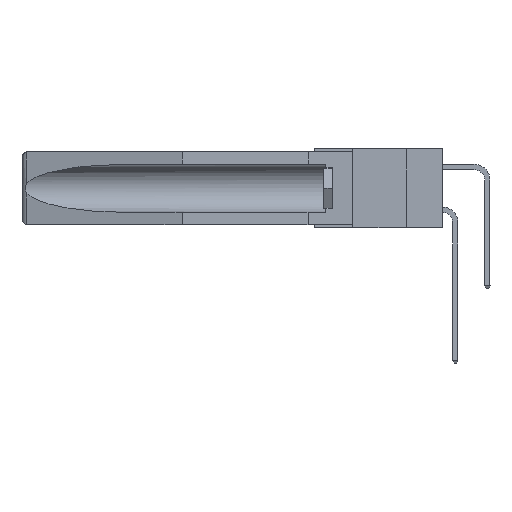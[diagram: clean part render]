
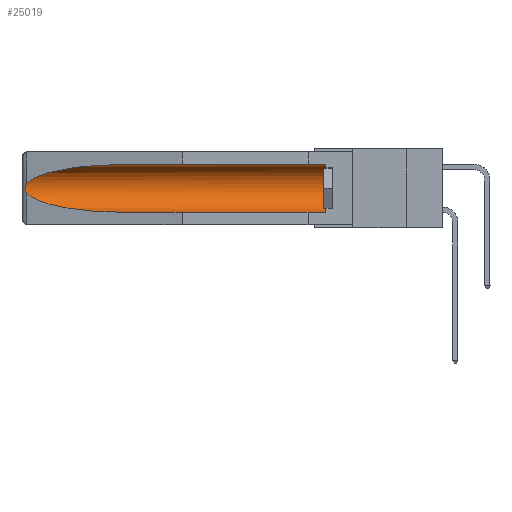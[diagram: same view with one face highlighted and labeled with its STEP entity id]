
A CAD part, left-side view. The second image highlights one B-rep face of the part: STEP entity #25019.
In plain terms, the highlighted cylindrical face has radius 2.857 mm (diameter 5.715 mm), a partial arc.
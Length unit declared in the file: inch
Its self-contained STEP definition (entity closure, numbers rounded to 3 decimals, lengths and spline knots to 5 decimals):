
#461 = CARTESIAN_POINT ( 'NONE',  ( 0.2675, 1.53308, -0.16763 ) ) ;
#484 =( BOUNDED_CURVE ( )  B_SPLINE_CURVE ( 3, ( #4614, #8867, #6759, #21605 ),
 .UNSPECIFIED., .F., .F. ) 
 B_SPLINE_CURVE_WITH_KNOTS ( ( 4, 4 ),
 ( 0.1948, 1.5708 ),
 .UNSPECIFIED. ) 
 CURVE ( )  GEOMETRIC_REPRESENTATION_ITEM ( )  RATIONAL_B_SPLINE_CURVE ( ( 1., 0.848, 0.848, 1. ) ) 
 REPRESENTATION_ITEM ( '' )  );
#530 = EDGE_CURVE ( 'NONE', #15714, #9848, #25866, .T. ) ;
#658 = CARTESIAN_POINT ( 'NONE',  ( 0.2673, 1.53269, -0.17917 ) ) ;
#691 = ORIENTED_EDGE ( 'NONE', *, *, #8976, .T. ) ;
#1311 = DIRECTION ( 'NONE',  ( 0., 0., 1. ) ) ;
#1348 =( BOUNDED_CURVE ( )  B_SPLINE_CURVE ( 3, ( #12060, #27133, #16369, #16184 ),
 .UNSPECIFIED., .F., .F. ) 
 B_SPLINE_CURVE_WITH_KNOTS ( ( 4, 4 ),
 ( 4.71239, 6.08839 ),
 .UNSPECIFIED. ) 
 CURVE ( )  GEOMETRIC_REPRESENTATION_ITEM ( )  RATIONAL_B_SPLINE_CURVE ( ( 1., 0.848, 0.848, 1. ) ) 
 REPRESENTATION_ITEM ( '' )  );
#1919 = DIRECTION ( 'NONE',  ( 0., 1., 0. ) ) ;
#3655 = CARTESIAN_POINT ( 'NONE',  ( 0.155, 1.07973, -0.284 ) ) ;
#4331 = VERTEX_POINT ( 'NONE', #21140 ) ;
#4614 = CARTESIAN_POINT ( 'NONE',  ( 0.26537, 1.52718, -0.19328 ) ) ;
#5009 = CARTESIAN_POINT ( 'NONE',  ( 0.26537, 1.52718, -0.19328 ) ) ;
#6759 = CARTESIAN_POINT ( 'NONE',  ( 0.21114, 1.30732, -0.284 ) ) ;
#6954 = ORIENTED_EDGE ( 'NONE', *, *, #23586, .T. ) ;
#7066 = CARTESIAN_POINT ( 'NONE',  ( 0.26597, 1.52961, -0.15275 ) ) ;
#7181 = FACE_OUTER_BOUND ( 'NONE', #10859, .T. ) ;
#7915 = CARTESIAN_POINT ( 'NONE',  ( 0.155, 0.126, -0.1715 ) ) ;
#8641 = ORIENTED_EDGE ( 'NONE', *, *, #11022, .F. ) ;
#8867 = CARTESIAN_POINT ( 'NONE',  ( 0.25451, 1.48313, -0.24835 ) ) ;
#8976 = EDGE_CURVE ( 'NONE', #9848, #22219, #484, .T. ) ;
#9036 = VERTEX_POINT ( 'NONE', #23087 ) ;
#9514 = CARTESIAN_POINT ( 'NONE',  ( 0.26654, 1.53092, -0.15636 ) ) ;
#9761 = CARTESIAN_POINT ( 'NONE',  ( 0.26537, 1.52718, -0.14972 ) ) ;
#9848 = VERTEX_POINT ( 'NONE', #20271 ) ;
#10859 = EDGE_LOOP ( 'NONE', ( #11641, #22779, #691, #8641, #15835, #6954 ) ) ;
#11022 = EDGE_CURVE ( 'NONE', #14541, #22219, #11442, .T. ) ;
#11214 = CARTESIAN_POINT ( 'NONE',  ( 0.26537, 1.52718, -0.14972 ) ) ;
#11442 = LINE ( 'NONE', #27418, #21535 ) ;
#11641 = ORIENTED_EDGE ( 'NONE', *, *, #22664, .T. ) ;
#12060 = CARTESIAN_POINT ( 'NONE',  ( 0.155, 1.07973, -0.059 ) ) ;
#12645 = DIRECTION ( 'NONE',  ( 0., 1., 0. ) ) ;
#12996 = LINE ( 'NONE', #13836, #20329 ) ;
#13836 = CARTESIAN_POINT ( 'NONE',  ( 0.155, -0.30754, -0.059 ) ) ;
#14188 = DIRECTION ( 'NONE',  ( 0., -1., 0. ) ) ;
#14329 = CARTESIAN_POINT ( 'NONE',  ( 0.155, 0.126, -0.284 ) ) ;
#14541 = VERTEX_POINT ( 'NONE', #14329 ) ;
#15714 = VERTEX_POINT ( 'NONE', #9761 ) ;
#15835 = ORIENTED_EDGE ( 'NONE', *, *, #17626, .T. ) ;
#16184 = CARTESIAN_POINT ( 'NONE',  ( 0.26537, 1.52718, -0.14972 ) ) ;
#16369 = CARTESIAN_POINT ( 'NONE',  ( 0.25451, 1.48313, -0.09465 ) ) ;
#16497 = AXIS2_PLACEMENT_3D ( 'NONE', #27538, #1919, #27629 ) ;
#17626 = EDGE_CURVE ( 'NONE', #14541, #4331, #23793, .T. ) ;
#17850 = CARTESIAN_POINT ( 'NONE',  ( 0.26597, 1.5296, -0.19026 ) ) ;
#20271 = CARTESIAN_POINT ( 'NONE',  ( 0.26537, 1.52718, -0.19328 ) ) ;
#20329 = VECTOR ( 'NONE', #22209, 39.37008 ) ;
#21140 = CARTESIAN_POINT ( 'NONE',  ( 0.155, 0.126, -0.059 ) ) ;
#21206 = AXIS2_PLACEMENT_3D ( 'NONE', #7915, #14188, #1311 ) ;
#21535 = VECTOR ( 'NONE', #12645, 39.37008 ) ;
#21605 = CARTESIAN_POINT ( 'NONE',  ( 0.155, 1.07973, -0.284 ) ) ;
#21643 = CYLINDRICAL_SURFACE ( 'NONE', #16497, 0.1125 ) ;
#22099 = CARTESIAN_POINT ( 'NONE',  ( 0.2673, 1.5327, -0.16383 ) ) ;
#22209 = DIRECTION ( 'NONE',  ( 0., 1., 0. ) ) ;
#22219 = VERTEX_POINT ( 'NONE', #3655 ) ;
#22664 = EDGE_CURVE ( 'NONE', #9036, #15714, #1348, .T. ) ;
#22779 = ORIENTED_EDGE ( 'NONE', *, *, #530, .T. ) ;
#23087 = CARTESIAN_POINT ( 'NONE',  ( 0.155, 1.07973, -0.059 ) ) ;
#23586 = EDGE_CURVE ( 'NONE', #4331, #9036, #12996, .T. ) ;
#23793 = CIRCLE ( 'NONE', #21206, 0.1125 ) ;
#24370 = CARTESIAN_POINT ( 'NONE',  ( 0.26655, 1.53094, -0.18657 ) ) ;
#25019 = ADVANCED_FACE ( 'NONE', ( #7181 ), #21643, .F. ) ;
#25866 = B_SPLINE_CURVE_WITH_KNOTS ( 'NONE', 3,
 ( #11214, #7066, #9514, #22099, #461, #26447, #658, #24370, #17850, #5009 ),
 .UNSPECIFIED., .F., .F.,
 ( 4, 2, 2, 2, 4 ),
 ( 0., 0.00029, 0.00058, 0.00087, 0.00117 ),
 .UNSPECIFIED. ) ;
#26447 = CARTESIAN_POINT ( 'NONE',  ( 0.2675, 1.53308, -0.17534 ) ) ;
#27133 = CARTESIAN_POINT ( 'NONE',  ( 0.21114, 1.30732, -0.059 ) ) ;
#27418 = CARTESIAN_POINT ( 'NONE',  ( 0.155, -0.30754, -0.284 ) ) ;
#27538 = CARTESIAN_POINT ( 'NONE',  ( 0.155, -0.30754, -0.1715 ) ) ;
#27629 = DIRECTION ( 'NONE',  ( 0., 0., 1. ) ) ;
